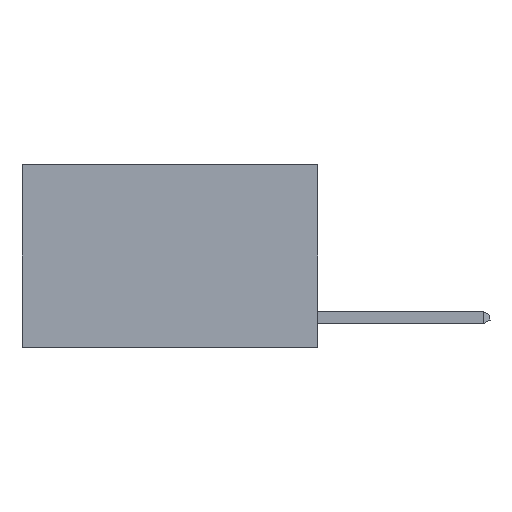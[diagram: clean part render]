
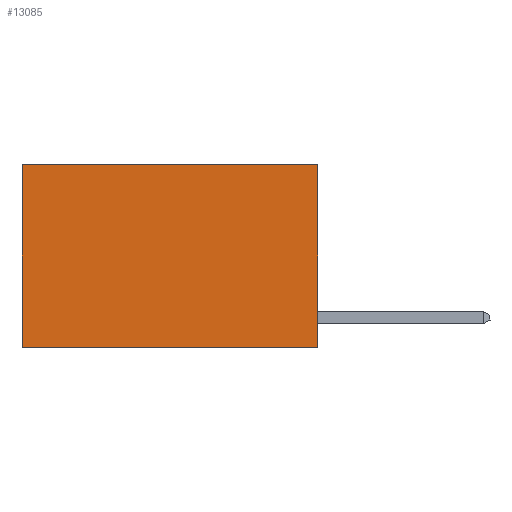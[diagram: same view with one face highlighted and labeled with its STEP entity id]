
A CAD part, left-side view. The second image highlights one B-rep face of the part: STEP entity #13085.
In plain terms, the highlighted planar face has unit normal (-1, 0, 0).
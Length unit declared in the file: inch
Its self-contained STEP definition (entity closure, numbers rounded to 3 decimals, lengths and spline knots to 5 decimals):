
#465 = ORIENTED_EDGE ( 'NONE', *, *, #10851, .T. ) ;
#918 = CARTESIAN_POINT ( 'NONE',  ( 0.2625, 0., 0. ) ) ;
#1035 = CARTESIAN_POINT ( 'NONE',  ( 0.2625, 0., -0.37 ) ) ;
#2989 = VERTEX_POINT ( 'NONE', #11027 ) ;
#3030 = VERTEX_POINT ( 'NONE', #4265 ) ;
#3204 = DIRECTION ( 'NONE',  ( 0., 1., 0. ) ) ;
#4169 = EDGE_CURVE ( 'NONE', #2989, #3030, #11263, .T. ) ;
#4228 = CARTESIAN_POINT ( 'NONE',  ( 0.2625, 0., 0. ) ) ;
#4265 = CARTESIAN_POINT ( 'NONE',  ( 0.2625, 0.6, -0.37 ) ) ;
#4473 = LINE ( 'NONE', #7627, #10054 ) ;
#5136 = PLANE ( 'NONE',  #12448 ) ;
#6138 = EDGE_LOOP ( 'NONE', ( #10379, #9029, #12114, #465 ) ) ;
#6174 = DIRECTION ( 'NONE',  ( 0., 0., -1. ) ) ;
#6722 = LINE ( 'NONE', #12606, #9023 ) ;
#6980 = CARTESIAN_POINT ( 'NONE',  ( 0.2625, 0.6, 0. ) ) ;
#7627 = CARTESIAN_POINT ( 'NONE',  ( 0.2625, 0., 0. ) ) ;
#8082 = CARTESIAN_POINT ( 'NONE',  ( 0.2625, 0., 0. ) ) ;
#8420 = VERTEX_POINT ( 'NONE', #4228 ) ;
#9023 = VECTOR ( 'NONE', #10622, 39.37008 ) ;
#9029 = ORIENTED_EDGE ( 'NONE', *, *, #4169, .F. ) ;
#9187 = DIRECTION ( 'NONE',  ( 0., 0., -1. ) ) ;
#9583 = EDGE_CURVE ( 'NONE', #8420, #2989, #10017, .T. ) ;
#10017 = LINE ( 'NONE', #918, #11411 ) ;
#10054 = VECTOR ( 'NONE', #11510, 39.37008 ) ;
#10233 = EDGE_CURVE ( 'NONE', #11053, #3030, #6722, .T. ) ;
#10379 = ORIENTED_EDGE ( 'NONE', *, *, #10233, .T. ) ;
#10622 = DIRECTION ( 'NONE',  ( 0., 0., -1. ) ) ;
#10781 = FACE_OUTER_BOUND ( 'NONE', #6138, .T. ) ;
#10851 = EDGE_CURVE ( 'NONE', #8420, #11053, #4473, .T. ) ;
#10976 = VECTOR ( 'NONE', #3204, 39.37008 ) ;
#11027 = CARTESIAN_POINT ( 'NONE',  ( 0.2625, 0., -0.37 ) ) ;
#11053 = VERTEX_POINT ( 'NONE', #6980 ) ;
#11263 = LINE ( 'NONE', #1035, #10976 ) ;
#11411 = VECTOR ( 'NONE', #9187, 39.37008 ) ;
#11510 = DIRECTION ( 'NONE',  ( 0., 1., 0. ) ) ;
#12068 = DIRECTION ( 'NONE',  ( 1., 0., 0. ) ) ;
#12114 = ORIENTED_EDGE ( 'NONE', *, *, #9583, .F. ) ;
#12448 = AXIS2_PLACEMENT_3D ( 'NONE', #8082, #12068, #6174 ) ;
#12606 = CARTESIAN_POINT ( 'NONE',  ( 0.2625, 0.6, 0. ) ) ;
#13085 = ADVANCED_FACE ( 'NONE', ( #10781 ), #5136, .F. ) ;
